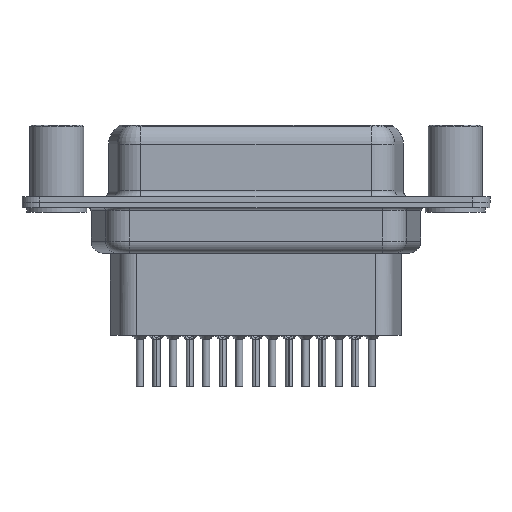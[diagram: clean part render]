
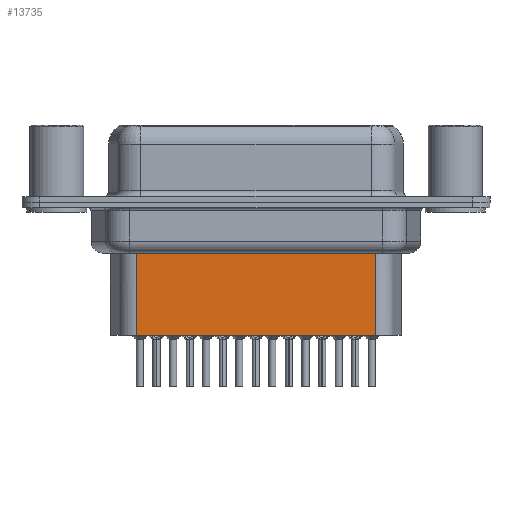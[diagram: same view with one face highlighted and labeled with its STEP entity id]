
A CAD part, front view. The second image highlights one B-rep face of the part: STEP entity #13735.
In plain terms, the highlighted planar face has unit normal (0, -1, 0).
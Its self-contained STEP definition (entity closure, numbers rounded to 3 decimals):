
#157 = DIRECTION ( 'NONE',  ( 0., -1., 0. ) ) ;
#170 = CARTESIAN_POINT ( 'NONE',  ( 26.619, -3.5, -4.097 ) ) ;
#237 = EDGE_CURVE ( 'NONE', #20500, #4496, #24160, .T. ) ;
#965 = DIRECTION ( 'NONE',  ( -1., 0., 0. ) ) ;
#1307 = CARTESIAN_POINT ( 'NONE',  ( 6.434, -3.5, -4.097 ) ) ;
#1639 = EDGE_CURVE ( 'NONE', #5204, #12652, #3172, .T. ) ;
#2648 = VECTOR ( 'NONE', #14245, 1000. ) ;
#3172 = LINE ( 'NONE', #1307, #3750 ) ;
#3348 = CARTESIAN_POINT ( 'NONE',  ( 6.681, -3.5, -3.1 ) ) ;
#3623 = CARTESIAN_POINT ( 'NONE',  ( 6.681, -3.5, -4.097 ) ) ;
#3750 = VECTOR ( 'NONE', #5173, 1000. ) ;
#4496 = VERTEX_POINT ( 'NONE', #22701 ) ;
#4598 = CARTESIAN_POINT ( 'NONE',  ( 26.619, -3.5, -11.15 ) ) ;
#4667 = ORIENTED_EDGE ( 'NONE', *, *, #17178, .F. ) ;
#5098 = ORIENTED_EDGE ( 'NONE', *, *, #1639, .T. ) ;
#5173 = DIRECTION ( 'NONE',  ( -1., 0., 0. ) ) ;
#5204 = VERTEX_POINT ( 'NONE', #170 ) ;
#6182 = PLANE ( 'NONE',  #18429 ) ;
#9012 = LINE ( 'NONE', #3348, #11525 ) ;
#9249 = EDGE_LOOP ( 'NONE', ( #4667, #5098, #16437, #14542 ) ) ;
#11525 = VECTOR ( 'NONE', #16645, 1000. ) ;
#11595 = DIRECTION ( 'NONE',  ( 1., 0., 0. ) ) ;
#11850 = FACE_OUTER_BOUND ( 'NONE', #9249, .T. ) ;
#12652 = VERTEX_POINT ( 'NONE', #3623 ) ;
#13735 = ADVANCED_FACE ( 'NONE', ( #11850 ), #6182, .T. ) ;
#14245 = DIRECTION ( 'NONE',  ( 0., 0., -1. ) ) ;
#14258 = CARTESIAN_POINT ( 'NONE',  ( 6.681, -3.5, -11.15 ) ) ;
#14542 = ORIENTED_EDGE ( 'NONE', *, *, #237, .F. ) ;
#15716 = CARTESIAN_POINT ( 'NONE',  ( 6.681, -3.5, -3.1 ) ) ;
#16437 = ORIENTED_EDGE ( 'NONE', *, *, #18908, .T. ) ;
#16645 = DIRECTION ( 'NONE',  ( 0., 0., -1. ) ) ;
#17178 = EDGE_CURVE ( 'NONE', #5204, #20500, #23389, .T. ) ;
#17664 = VECTOR ( 'NONE', #965, 1000. ) ;
#17760 = CARTESIAN_POINT ( 'NONE',  ( 26.619, -3.5, -3.1 ) ) ;
#18429 = AXIS2_PLACEMENT_3D ( 'NONE', #15716, #157, #11595 ) ;
#18908 = EDGE_CURVE ( 'NONE', #12652, #4496, #9012, .T. ) ;
#20500 = VERTEX_POINT ( 'NONE', #4598 ) ;
#22701 = CARTESIAN_POINT ( 'NONE',  ( 6.681, -3.5, -11.15 ) ) ;
#23389 = LINE ( 'NONE', #17760, #2648 ) ;
#24160 = LINE ( 'NONE', #14258, #17664 ) ;
